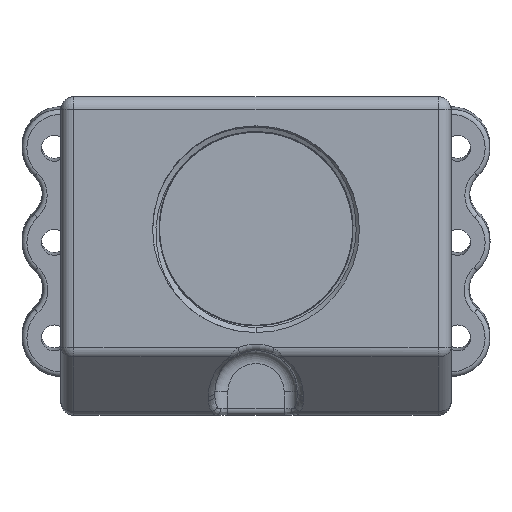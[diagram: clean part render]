
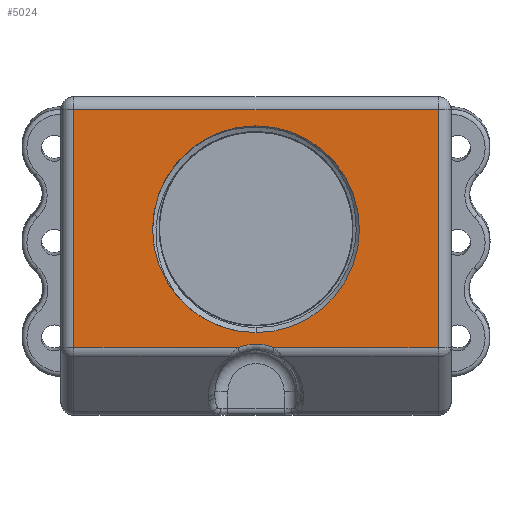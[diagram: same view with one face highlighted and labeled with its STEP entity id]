
A CAD part, top view. The second image highlights one B-rep face of the part: STEP entity #5024.
In plain terms, the highlighted planar face has unit normal (0, 0, 1).
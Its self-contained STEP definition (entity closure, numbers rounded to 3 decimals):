
#188=FACE_BOUND('',#1022,.T.);
#470=PLANE('',#5418);
#696=FACE_OUTER_BOUND('',#1021,.T.);
#1021=EDGE_LOOP('',(#3745,#3746,#3747,#3748,#3749,#3750));
#1022=EDGE_LOOP('',(#3751));
#1361=CIRCLE('',#5373,15.951);
#1371=CIRCLE('',#5391,7.35);
#1844=LINE('',#11523,#2122);
#1845=LINE('',#11525,#2123);
#1846=LINE('',#11527,#2124);
#1847=LINE('',#11529,#2125);
#1848=LINE('',#11530,#2126);
#2122=VECTOR('',#6150,10.);
#2123=VECTOR('',#6151,10.);
#2124=VECTOR('',#6152,10.);
#2125=VECTOR('',#6153,10.);
#2126=VECTOR('',#6154,10.);
#2410=VERTEX_POINT('',#8687);
#2427=VERTEX_POINT('',#11271);
#2429=VERTEX_POINT('',#11285);
#2450=VERTEX_POINT('',#11522);
#2451=VERTEX_POINT('',#11524);
#2452=VERTEX_POINT('',#11526);
#2453=VERTEX_POINT('',#11528);
#2883=EDGE_CURVE('',#2410,#2410,#1361,.T.);
#2914=EDGE_CURVE('',#2429,#2427,#1371,.T.);
#2950=EDGE_CURVE('',#2450,#2429,#1844,.T.);
#2951=EDGE_CURVE('',#2451,#2450,#1845,.T.);
#2952=EDGE_CURVE('',#2452,#2451,#1846,.T.);
#2953=EDGE_CURVE('',#2453,#2452,#1847,.T.);
#2954=EDGE_CURVE('',#2427,#2453,#1848,.T.);
#3745=ORIENTED_EDGE('',*,*,#2914,.F.);
#3746=ORIENTED_EDGE('',*,*,#2950,.F.);
#3747=ORIENTED_EDGE('',*,*,#2951,.F.);
#3748=ORIENTED_EDGE('',*,*,#2952,.F.);
#3749=ORIENTED_EDGE('',*,*,#2953,.F.);
#3750=ORIENTED_EDGE('',*,*,#2954,.F.);
#3751=ORIENTED_EDGE('',*,*,#2883,.T.);
#5024=ADVANCED_FACE('',(#696,#188),#470,.T.);
#5373=AXIS2_PLACEMENT_3D('',#8689,#6044,#6045);
#5391=AXIS2_PLACEMENT_3D('',#11287,#6082,#6083);
#5418=AXIS2_PLACEMENT_3D('',#11521,#6148,#6149);
#6044=DIRECTION('center_axis',(0.,0.,-1.));
#6045=DIRECTION('ref_axis',(-1.,0.,0.));
#6082=DIRECTION('center_axis',(0.,0.,1.));
#6083=DIRECTION('ref_axis',(-0.385,0.923,0.));
#6148=DIRECTION('center_axis',(0.,0.,1.));
#6149=DIRECTION('ref_axis',(1.,0.,0.));
#6150=DIRECTION('',(-1.,0.,0.));
#6151=DIRECTION('',(0.,-1.,0.));
#6152=DIRECTION('',(1.,0.,0.));
#6153=DIRECTION('',(0.,1.,0.));
#6154=DIRECTION('',(-1.,0.,0.));
#8687=CARTESIAN_POINT('',(15.951,-20.54,285.));
#8689=CARTESIAN_POINT('Origin',(0.,-20.54,285.));
#11271=CARTESIAN_POINT('',(-2.83,-38.819,285.));
#11285=CARTESIAN_POINT('',(2.83,-38.819,285.));
#11287=CARTESIAN_POINT('Origin',(0.,-45.602,
285.));
#11521=CARTESIAN_POINT('Origin',(0.412,-20.932,285.));
#11522=CARTESIAN_POINT('',(28.1,-38.819,285.));
#11523=CARTESIAN_POINT('',(5.8,-38.819,285.));
#11524=CARTESIAN_POINT('',(28.1,-2.086,285.));
#11525=CARTESIAN_POINT('',(28.1,-21.538,285.));
#11526=CARTESIAN_POINT('',(-28.1,-2.086,285.));
#11527=CARTESIAN_POINT('',(8.05,-2.086,285.));
#11528=CARTESIAN_POINT('',(-28.1,-38.819,285.));
#11529=CARTESIAN_POINT('',(-28.1,-21.538,285.));
#11530=CARTESIAN_POINT('',(5.8,-38.819,285.));
